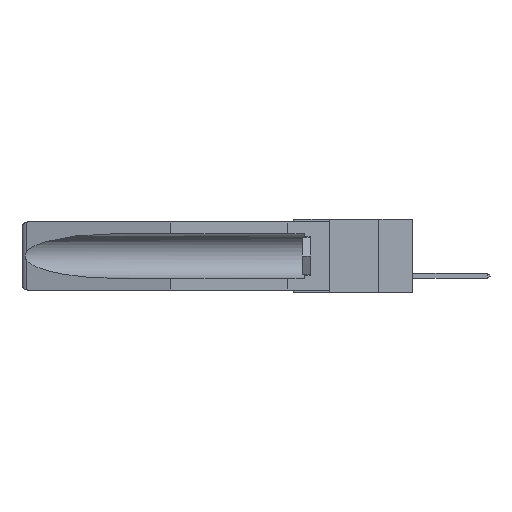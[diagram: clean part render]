
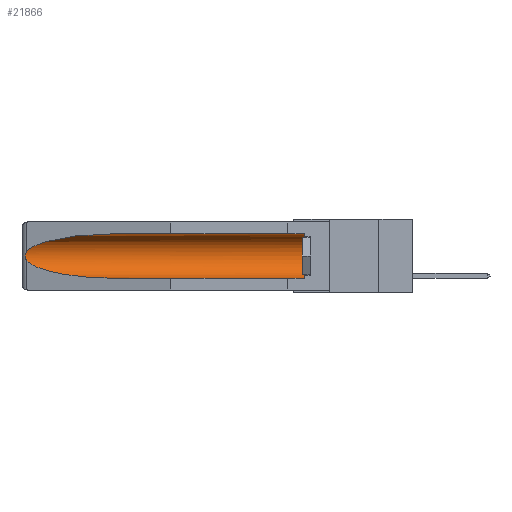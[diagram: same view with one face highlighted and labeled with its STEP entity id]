
A CAD part, left-side view. The second image highlights one B-rep face of the part: STEP entity #21866.
In plain terms, the highlighted cylindrical face has radius 2.857 mm (diameter 5.715 mm), a partial arc.
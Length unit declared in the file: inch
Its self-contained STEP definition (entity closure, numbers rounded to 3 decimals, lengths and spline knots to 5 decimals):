
#1240 = DIRECTION ( 'NONE',  ( 0., 1., 0. ) ) ;
#1662 = LINE ( 'NONE', #27220, #15190 ) ;
#1868 = EDGE_CURVE ( 'NONE', #27823, #11994, #1662, .T. ) ;
#2338 = CARTESIAN_POINT ( 'NONE',  ( 0.26537, 1.52718, -0.14972 ) ) ;
#2596 = LINE ( 'NONE', #30542, #27337 ) ;
#2606 = CARTESIAN_POINT ( 'NONE',  ( 0.26537, 1.52718, -0.19328 ) ) ;
#2695 = FACE_OUTER_BOUND ( 'NONE', #27365, .T. ) ;
#2793 = AXIS2_PLACEMENT_3D ( 'NONE', #16032, #1240, #18504 ) ;
#3111 = ORIENTED_EDGE ( 'NONE', *, *, #22150, .T. ) ;
#3461 = EDGE_CURVE ( 'NONE', #25198, #17550, #21844, .T. ) ;
#3648 = CARTESIAN_POINT ( 'NONE',  ( 0.155, 0.126, -0.1715 ) ) ;
#3729 = CARTESIAN_POINT ( 'NONE',  ( 0.155, 1.07973, -0.284 ) ) ;
#4102 = CARTESIAN_POINT ( 'NONE',  ( 0.26597, 1.52961, -0.15275 ) ) ;
#5086 = CARTESIAN_POINT ( 'NONE',  ( 0.21114, 1.30732, -0.284 ) ) ;
#5196 =( BOUNDED_CURVE ( )  B_SPLINE_CURVE ( 3, ( #2606, #19895, #5086, #22376 ),
 .UNSPECIFIED., .F., .T. ) 
 B_SPLINE_CURVE_WITH_KNOTS ( ( 4, 4 ),
 ( 0.1948, 1.5708 ),
 .UNSPECIFIED. ) 
 CURVE ( )  GEOMETRIC_REPRESENTATION_ITEM ( )  RATIONAL_B_SPLINE_CURVE ( ( 1., 0.848, 0.848, 1. ) ) 
 REPRESENTATION_ITEM ( '' )  );
#6194 = ORIENTED_EDGE ( 'NONE', *, *, #23804, .T. ) ;
#6381 = EDGE_CURVE ( 'NONE', #27823, #11260, #26621, .T. ) ;
#6557 = CARTESIAN_POINT ( 'NONE',  ( 0.155, 0.126, -0.059 ) ) ;
#6697 = CARTESIAN_POINT ( 'NONE',  ( 0.2675, 1.53308, -0.16763 ) ) ;
#8046 = CARTESIAN_POINT ( 'NONE',  ( 0.155, 0.126, -0.284 ) ) ;
#8968 =( BOUNDED_CURVE ( )  B_SPLINE_CURVE ( 3, ( #11792, #9098, #14088, #31361 ),
 .UNSPECIFIED., .F., .F. ) 
 B_SPLINE_CURVE_WITH_KNOTS ( ( 4, 4 ),
 ( 4.71239, 6.08839 ),
 .UNSPECIFIED. ) 
 CURVE ( )  GEOMETRIC_REPRESENTATION_ITEM ( )  RATIONAL_B_SPLINE_CURVE ( ( 1., 0.848, 0.848, 1. ) ) 
 REPRESENTATION_ITEM ( '' )  );
#9098 = CARTESIAN_POINT ( 'NONE',  ( 0.21114, 1.30732, -0.059 ) ) ;
#9966 = ORIENTED_EDGE ( 'NONE', *, *, #6381, .T. ) ;
#10783 = DIRECTION ( 'NONE',  ( 0., 1., 0. ) ) ;
#11260 = VERTEX_POINT ( 'NONE', #6557 ) ;
#11470 = CARTESIAN_POINT ( 'NONE',  ( 0.2673, 1.5327, -0.16383 ) ) ;
#11792 = CARTESIAN_POINT ( 'NONE',  ( 0.155, 1.07973, -0.059 ) ) ;
#11994 = VERTEX_POINT ( 'NONE', #3729 ) ;
#13750 = CARTESIAN_POINT ( 'NONE',  ( 0.26537, 1.52718, -0.19328 ) ) ;
#13860 = CARTESIAN_POINT ( 'NONE',  ( 0.26537, 1.52718, -0.14972 ) ) ;
#14088 = CARTESIAN_POINT ( 'NONE',  ( 0.25451, 1.48313, -0.09465 ) ) ;
#15190 = VECTOR ( 'NONE', #27547, 39.37008 ) ;
#15767 = AXIS2_PLACEMENT_3D ( 'NONE', #3648, #18698, #31228 ) ;
#16032 = CARTESIAN_POINT ( 'NONE',  ( 0.155, -0.30754, -0.1715 ) ) ;
#16464 = CARTESIAN_POINT ( 'NONE',  ( 0.155, 1.07973, -0.059 ) ) ;
#17550 = VERTEX_POINT ( 'NONE', #29432 ) ;
#18193 = EDGE_CURVE ( 'NONE', #11260, #22853, #2596, .T. ) ;
#18504 = DIRECTION ( 'NONE',  ( 0., 0., 1. ) ) ;
#18698 = DIRECTION ( 'NONE',  ( 0., -1., 0. ) ) ;
#19895 = CARTESIAN_POINT ( 'NONE',  ( 0.25451, 1.48313, -0.24835 ) ) ;
#20194 = ORIENTED_EDGE ( 'NONE', *, *, #3461, .T. ) ;
#21401 = CARTESIAN_POINT ( 'NONE',  ( 0.26654, 1.53092, -0.15636 ) ) ;
#21506 = CARTESIAN_POINT ( 'NONE',  ( 0.2675, 1.53308, -0.17534 ) ) ;
#21844 = B_SPLINE_CURVE_WITH_KNOTS ( 'NONE', 3,
 ( #13860, #4102, #21401, #11470, #6697, #21506, #28736, #26048, #26368, #13750 ),
 .UNSPECIFIED., .F., .F.,
 ( 4, 2, 2, 2, 4 ),
 ( 0., 0.00029, 0.00058, 0.00087, 0.00117 ),
 .UNSPECIFIED. ) ;
#21866 = ADVANCED_FACE ( 'NONE', ( #2695 ), #30503, .F. ) ;
#22150 = EDGE_CURVE ( 'NONE', #17550, #11994, #5196, .T. ) ;
#22237 = ORIENTED_EDGE ( 'NONE', *, *, #18193, .T. ) ;
#22376 = CARTESIAN_POINT ( 'NONE',  ( 0.155, 1.07973, -0.284 ) ) ;
#22853 = VERTEX_POINT ( 'NONE', #16464 ) ;
#23804 = EDGE_CURVE ( 'NONE', #22853, #25198, #8968, .T. ) ;
#25198 = VERTEX_POINT ( 'NONE', #2338 ) ;
#26048 = CARTESIAN_POINT ( 'NONE',  ( 0.26655, 1.53094, -0.18657 ) ) ;
#26368 = CARTESIAN_POINT ( 'NONE',  ( 0.26597, 1.5296, -0.19026 ) ) ;
#26621 = CIRCLE ( 'NONE', #15767, 0.1125 ) ;
#27220 = CARTESIAN_POINT ( 'NONE',  ( 0.155, -0.30754, -0.284 ) ) ;
#27337 = VECTOR ( 'NONE', #10783, 39.37008 ) ;
#27365 = EDGE_LOOP ( 'NONE', ( #6194, #20194, #3111, #31208, #9966, #22237 ) ) ;
#27547 = DIRECTION ( 'NONE',  ( 0., 1., 0. ) ) ;
#27823 = VERTEX_POINT ( 'NONE', #8046 ) ;
#28736 = CARTESIAN_POINT ( 'NONE',  ( 0.2673, 1.53269, -0.17917 ) ) ;
#29432 = CARTESIAN_POINT ( 'NONE',  ( 0.26537, 1.52718, -0.19328 ) ) ;
#30503 = CYLINDRICAL_SURFACE ( 'NONE', #2793, 0.1125 ) ;
#30542 = CARTESIAN_POINT ( 'NONE',  ( 0.155, -0.30754, -0.059 ) ) ;
#31208 = ORIENTED_EDGE ( 'NONE', *, *, #1868, .F. ) ;
#31228 = DIRECTION ( 'NONE',  ( 0., 0., 1. ) ) ;
#31361 = CARTESIAN_POINT ( 'NONE',  ( 0.26537, 1.52718, -0.14972 ) ) ;
